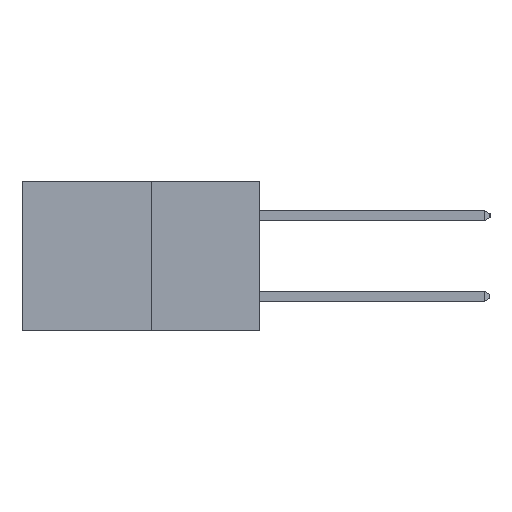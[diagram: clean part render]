
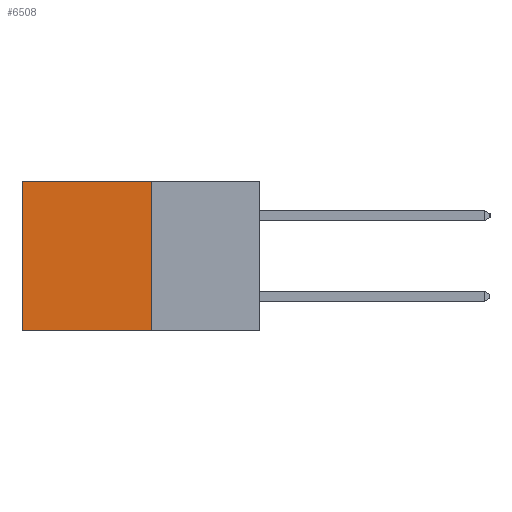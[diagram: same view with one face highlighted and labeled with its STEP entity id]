
A CAD part, left-side view. The second image highlights one B-rep face of the part: STEP entity #6508.
In plain terms, the highlighted planar face has unit normal (-1, 0, 0).
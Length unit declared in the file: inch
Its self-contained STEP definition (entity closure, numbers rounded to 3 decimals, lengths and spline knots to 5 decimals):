
#13 = DIRECTION ( 'NONE',  ( 0., 0., -1. ) ) ;
#610 = CARTESIAN_POINT ( 'NONE',  ( 0.277, 0.27, 0. ) ) ;
#736 = VECTOR ( 'NONE', #4960, 39.37008 ) ;
#1211 = ORIENTED_EDGE ( 'NONE', *, *, #7870, .F. ) ;
#1718 = CARTESIAN_POINT ( 'NONE',  ( 0.277, 0.27, 0. ) ) ;
#1786 = EDGE_CURVE ( 'NONE', #2305, #3382, #8708, .T. ) ;
#1921 = CARTESIAN_POINT ( 'NONE',  ( 0.277, 0.27, -0.37 ) ) ;
#2305 = VERTEX_POINT ( 'NONE', #610 ) ;
#2733 = LINE ( 'NONE', #3512, #9558 ) ;
#3382 = VERTEX_POINT ( 'NONE', #5507 ) ;
#3512 = CARTESIAN_POINT ( 'NONE',  ( 0.277, 0.27, -0.37 ) ) ;
#3615 = CARTESIAN_POINT ( 'NONE',  ( 0.277, 0.59, -0.37 ) ) ;
#3716 = VECTOR ( 'NONE', #5557, 39.37008 ) ;
#4057 = CARTESIAN_POINT ( 'NONE',  ( 0.277, 0.59, -0.37 ) ) ;
#4702 = FACE_OUTER_BOUND ( 'NONE', #7868, .T. ) ;
#4960 = DIRECTION ( 'NONE',  ( 0., 0., -1. ) ) ;
#5331 = DIRECTION ( 'NONE',  ( 0., 1., 0. ) ) ;
#5395 = EDGE_CURVE ( 'NONE', #6315, #6443, #10587, .T. ) ;
#5507 = CARTESIAN_POINT ( 'NONE',  ( 0.277, 0.27, -0.37 ) ) ;
#5537 = DIRECTION ( 'NONE',  ( 1., 0., 0. ) ) ;
#5557 = DIRECTION ( 'NONE',  ( 0., 0., -1. ) ) ;
#6315 = VERTEX_POINT ( 'NONE', #7053 ) ;
#6443 = VERTEX_POINT ( 'NONE', #3615 ) ;
#6508 = ADVANCED_FACE ( 'NONE', ( #4702 ), #9080, .F. ) ;
#7053 = CARTESIAN_POINT ( 'NONE',  ( 0.277, 0.59, 0. ) ) ;
#7868 = EDGE_LOOP ( 'NONE', ( #10486, #1211, #8400, #10732 ) ) ;
#7870 = EDGE_CURVE ( 'NONE', #3382, #6443, #2733, .T. ) ;
#7974 = DIRECTION ( 'NONE',  ( 0., 1., 0. ) ) ;
#8201 = LINE ( 'NONE', #1718, #10557 ) ;
#8400 = ORIENTED_EDGE ( 'NONE', *, *, #1786, .F. ) ;
#8708 = LINE ( 'NONE', #9315, #3716 ) ;
#9080 = PLANE ( 'NONE',  #9885 ) ;
#9315 = CARTESIAN_POINT ( 'NONE',  ( 0.277, 0.27, -0.37 ) ) ;
#9558 = VECTOR ( 'NONE', #7974, 39.37008 ) ;
#9885 = AXIS2_PLACEMENT_3D ( 'NONE', #1921, #5537, #13 ) ;
#10486 = ORIENTED_EDGE ( 'NONE', *, *, #5395, .T. ) ;
#10557 = VECTOR ( 'NONE', #5331, 39.37008 ) ;
#10587 = LINE ( 'NONE', #4057, #736 ) ;
#10732 = ORIENTED_EDGE ( 'NONE', *, *, #11429, .T. ) ;
#11429 = EDGE_CURVE ( 'NONE', #2305, #6315, #8201, .T. ) ;
